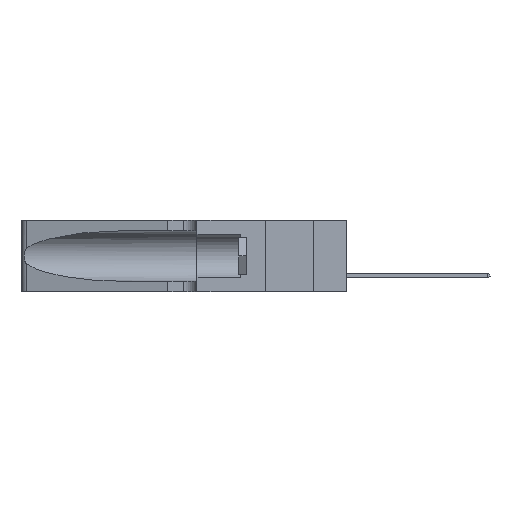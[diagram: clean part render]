
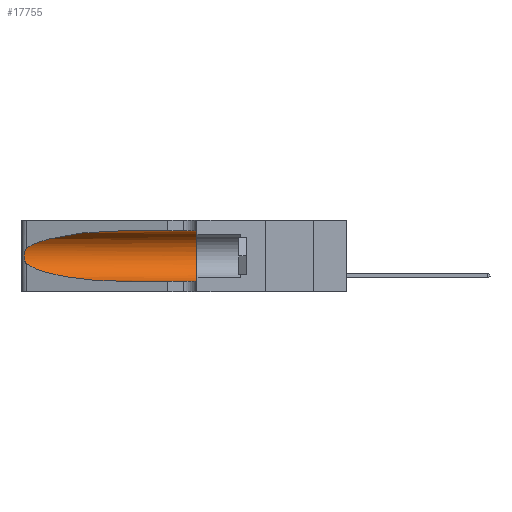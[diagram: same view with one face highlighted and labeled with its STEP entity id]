
A CAD part, left-side view. The second image highlights one B-rep face of the part: STEP entity #17755.
In plain terms, the highlighted cylindrical face has radius 3.308 mm (diameter 6.617 mm), a partial arc.
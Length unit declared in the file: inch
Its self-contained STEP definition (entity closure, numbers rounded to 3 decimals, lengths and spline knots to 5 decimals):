
#1783 = CARTESIAN_POINT ( 'NONE',  ( 0.25555, 1.22993, 0.14849 ) ) ;
#2073 = CARTESIAN_POINT ( 'NONE',  ( 0.26018, 1.23835, 0.19895 ) ) ;
#2362 = B_SPLINE_CURVE_WITH_KNOTS ( 'NONE', 3,
 ( #25467, #35980, #22576, #25621, #39434, #2073, #4943, #36134, #8981, #39734, #8833, #32973, #1783, #12413 ),
 .UNSPECIFIED., .F., .F.,
 ( 4, 2, 2, 2, 2, 2, 4 ),
 ( 0., 0.00027, 0.00053, 0.00107, 0.0016, 0.00187, 0.00214 ),
 .UNSPECIFIED. ) ;
#3198 =( BOUNDED_CURVE ( )  B_SPLINE_CURVE ( 3, ( #12554, #19743, #9401, #16458 ),
 .UNSPECIFIED., .F., .F. ) 
 B_SPLINE_CURVE_WITH_KNOTS ( ( 4, 4 ),
 ( 3.44316, 4.71239 ),
 .UNSPECIFIED. ) 
 CURVE ( )  GEOMETRIC_REPRESENTATION_ITEM ( )  RATIONAL_B_SPLINE_CURVE ( ( 1., 0.87, 0.87, 1. ) ) 
 REPRESENTATION_ITEM ( '' )  );
#3540 = ORIENTED_EDGE ( 'NONE', *, *, #41785, .T. ) ;
#3729 = VERTEX_POINT ( 'NONE', #8191 ) ;
#4202 = EDGE_CURVE ( 'NONE', #3729, #21271, #7710, .T. ) ;
#4605 = VERTEX_POINT ( 'NONE', #33806 ) ;
#4943 = CARTESIAN_POINT ( 'NONE',  ( 0.26075, 1.23896, 0.19203 ) ) ;
#5156 = CARTESIAN_POINT ( 'NONE',  ( 0.1305, 1.61858, 0.185 ) ) ;
#6400 = VERTEX_POINT ( 'NONE', #26757 ) ;
#7710 = LINE ( 'NONE', #15131, #12509 ) ;
#8191 = CARTESIAN_POINT ( 'NONE',  ( 0.1305, 0.72297, 0.31525 ) ) ;
#8833 = CARTESIAN_POINT ( 'NONE',  ( 0.25789, 1.23486, 0.15765 ) ) ;
#8981 = CARTESIAN_POINT ( 'NONE',  ( 0.26017, 1.23833, 0.17102 ) ) ;
#9401 = CARTESIAN_POINT ( 'NONE',  ( 0.18966, 0.96281, 0.05475 ) ) ;
#11071 = CARTESIAN_POINT ( 'NONE',  ( 0.25487, 1.22718, 0.22369 ) ) ;
#12413 = CARTESIAN_POINT ( 'NONE',  ( 0.25487, 1.22718, 0.14631 ) ) ;
#12509 = VECTOR ( 'NONE', #35123, 39.37008 ) ;
#12554 = CARTESIAN_POINT ( 'NONE',  ( 0.25487, 1.22718, 0.14631 ) ) ;
#13601 = DIRECTION ( 'NONE',  ( 0., -1., 0. ) ) ;
#13644 = ORIENTED_EDGE ( 'NONE', *, *, #33884, .T. ) ;
#13966 = AXIS2_PLACEMENT_3D ( 'NONE', #5156, #42500, #21914 ) ;
#14306 = EDGE_CURVE ( 'NONE', #21271, #20530, #34949, .T. ) ;
#14958 = ORIENTED_EDGE ( 'NONE', *, *, #29141, .T. ) ;
#15120 = CARTESIAN_POINT ( 'NONE',  ( 0.1305, 0.35, 0.185 ) ) ;
#15131 = CARTESIAN_POINT ( 'NONE',  ( 0.1305, 1.61858, 0.31525 ) ) ;
#16458 = CARTESIAN_POINT ( 'NONE',  ( 0.1305, 0.72297, 0.05475 ) ) ;
#17059 = AXIS2_PLACEMENT_3D ( 'NONE', #15120, #39571, #29052 ) ;
#17755 = ADVANCED_FACE ( 'NONE', ( #33106 ), #30963, .F. ) ;
#17910 = VERTEX_POINT ( 'NONE', #33327 ) ;
#19344 = EDGE_LOOP ( 'NONE', ( #13644, #26403, #3540, #14958, #31542, #29644 ) ) ;
#19743 = CARTESIAN_POINT ( 'NONE',  ( 0.2373, 1.15595, 0.08982 ) ) ;
#20530 = VERTEX_POINT ( 'NONE', #36711 ) ;
#21271 = VERTEX_POINT ( 'NONE', #27332 ) ;
#21546 = CARTESIAN_POINT ( 'NONE',  ( 0.18966, 0.96281, 0.31525 ) ) ;
#21914 = DIRECTION ( 'NONE',  ( 0., 0., -1. ) ) ;
#22576 = CARTESIAN_POINT ( 'NONE',  ( 0.25639, 1.23184, 0.21858 ) ) ;
#24697 = CARTESIAN_POINT ( 'NONE',  ( 0.2373, 1.15595, 0.28018 ) ) ;
#25467 = CARTESIAN_POINT ( 'NONE',  ( 0.25487, 1.22718, 0.22369 ) ) ;
#25621 = CARTESIAN_POINT ( 'NONE',  ( 0.25787, 1.23484, 0.2124 ) ) ;
#26380 = VECTOR ( 'NONE', #13601, 39.37008 ) ;
#26403 = ORIENTED_EDGE ( 'NONE', *, *, #32045, .T. ) ;
#26757 = CARTESIAN_POINT ( 'NONE',  ( 0.1305, 0.72297, 0.05475 ) ) ;
#27332 = CARTESIAN_POINT ( 'NONE',  ( 0.1305, 0.35, 0.31525 ) ) ;
#28442 =( BOUNDED_CURVE ( )  B_SPLINE_CURVE ( 3, ( #41987, #21546, #24697, #11071 ),
 .UNSPECIFIED., .F., .T. ) 
 B_SPLINE_CURVE_WITH_KNOTS ( ( 4, 4 ),
 ( 1.5708, 2.84003 ),
 .UNSPECIFIED. ) 
 CURVE ( )  GEOMETRIC_REPRESENTATION_ITEM ( )  RATIONAL_B_SPLINE_CURVE ( ( 1., 0.87, 0.87, 1. ) ) 
 REPRESENTATION_ITEM ( '' )  );
#29052 = DIRECTION ( 'NONE',  ( 0., 0., 1. ) ) ;
#29141 = EDGE_CURVE ( 'NONE', #6400, #20530, #33932, .T. ) ;
#29644 = ORIENTED_EDGE ( 'NONE', *, *, #4202, .F. ) ;
#30963 = CYLINDRICAL_SURFACE ( 'NONE', #13966, 0.13025 ) ;
#31542 = ORIENTED_EDGE ( 'NONE', *, *, #14306, .F. ) ;
#32045 = EDGE_CURVE ( 'NONE', #4605, #17910, #2362, .T. ) ;
#32973 = CARTESIAN_POINT ( 'NONE',  ( 0.25639, 1.23186, 0.15144 ) ) ;
#33106 = FACE_OUTER_BOUND ( 'NONE', #19344, .T. ) ;
#33327 = CARTESIAN_POINT ( 'NONE',  ( 0.25487, 1.22718, 0.14631 ) ) ;
#33806 = CARTESIAN_POINT ( 'NONE',  ( 0.25487, 1.22718, 0.22369 ) ) ;
#33884 = EDGE_CURVE ( 'NONE', #3729, #4605, #28442, .T. ) ;
#33932 = LINE ( 'NONE', #37760, #26380 ) ;
#34949 = CIRCLE ( 'NONE', #17059, 0.13025 ) ;
#35123 = DIRECTION ( 'NONE',  ( 0., -1., 0. ) ) ;
#35980 = CARTESIAN_POINT ( 'NONE',  ( 0.25555, 1.22994, 0.2215 ) ) ;
#36134 = CARTESIAN_POINT ( 'NONE',  ( 0.26075, 1.23896, 0.178 ) ) ;
#36711 = CARTESIAN_POINT ( 'NONE',  ( 0.1305, 0.35, 0.05475 ) ) ;
#37760 = CARTESIAN_POINT ( 'NONE',  ( 0.1305, 1.61858, 0.05475 ) ) ;
#39434 = CARTESIAN_POINT ( 'NONE',  ( 0.25854, 1.2359, 0.20912 ) ) ;
#39571 = DIRECTION ( 'NONE',  ( 0., 1., 0. ) ) ;
#39734 = CARTESIAN_POINT ( 'NONE',  ( 0.25856, 1.23593, 0.16098 ) ) ;
#41785 = EDGE_CURVE ( 'NONE', #17910, #6400, #3198, .T. ) ;
#41987 = CARTESIAN_POINT ( 'NONE',  ( 0.1305, 0.72297, 0.31525 ) ) ;
#42500 = DIRECTION ( 'NONE',  ( 0., -1., 0. ) ) ;
